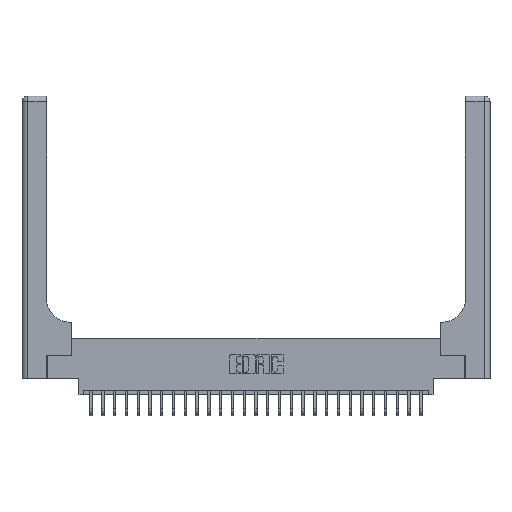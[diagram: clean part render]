
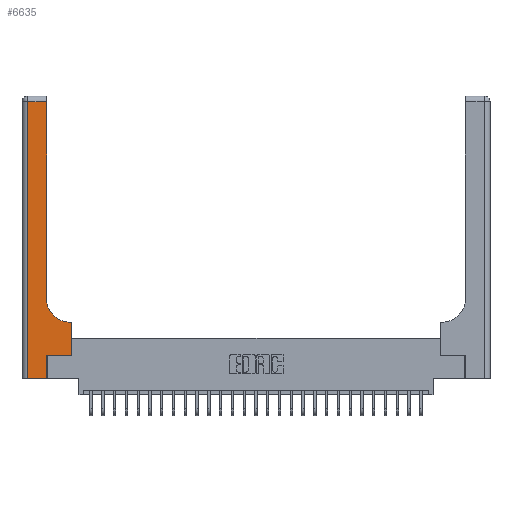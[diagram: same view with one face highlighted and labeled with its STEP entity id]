
A CAD part, top view. The second image highlights one B-rep face of the part: STEP entity #6635.
In plain terms, the highlighted planar face has unit normal (0, 0, 1).
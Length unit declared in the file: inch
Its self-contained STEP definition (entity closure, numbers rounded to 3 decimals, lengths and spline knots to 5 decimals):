
#686 = VECTOR ( 'NONE', #10712, 39.37008 ) ;
#997 = VERTEX_POINT ( 'NONE', #21001 ) ;
#1038 = EDGE_CURVE ( 'NONE', #25096, #25531, #8408, .T. ) ;
#1556 = LINE ( 'NONE', #10293, #5344 ) ;
#1730 = VERTEX_POINT ( 'NONE', #16154 ) ;
#1779 = CARTESIAN_POINT ( 'NONE',  ( 0., 2.94, 0.37 ) ) ;
#2214 = VERTEX_POINT ( 'NONE', #14119 ) ;
#2800 = ORIENTED_EDGE ( 'NONE', *, *, #14991, .T. ) ;
#3095 = VERTEX_POINT ( 'NONE', #4101 ) ;
#3140 = PLANE ( 'NONE',  #20049 ) ;
#3275 = FACE_OUTER_BOUND ( 'NONE', #4029, .T. ) ;
#4029 = EDGE_LOOP ( 'NONE', ( #19312, #25460, #20904, #24390, #14904, #2800, #17983, #15083, #19964 ) ) ;
#4101 = CARTESIAN_POINT ( 'NONE',  ( 0.06, 0., 0.37 ) ) ;
#4156 = DIRECTION ( 'NONE',  ( 0., 1., 0. ) ) ;
#4388 = VECTOR ( 'NONE', #26539, 39.37008 ) ;
#4410 = CARTESIAN_POINT ( 'NONE',  ( 0.06, 3., 0.37 ) ) ;
#4793 = CARTESIAN_POINT ( 'NONE',  ( 0.26, 0.85, 0.37 ) ) ;
#5344 = VECTOR ( 'NONE', #25563, 39.37008 ) ;
#5503 = VECTOR ( 'NONE', #4156, 39.37008 ) ;
#6266 = DIRECTION ( 'NONE',  ( 0., -1., 0. ) ) ;
#6635 = ADVANCED_FACE ( 'NONE', ( #3275 ), #3140, .F. ) ;
#8408 = LINE ( 'NONE', #23698, #686 ) ;
#8891 = LINE ( 'NONE', #23746, #5503 ) ;
#9444 = DIRECTION ( 'NONE',  ( 0., 0., -1. ) ) ;
#9636 = CARTESIAN_POINT ( 'NONE',  ( 0.51, 0.6, 0.37 ) ) ;
#10293 = CARTESIAN_POINT ( 'NONE',  ( 0.26, 0.6, 0.37 ) ) ;
#10712 = DIRECTION ( 'NONE',  ( 0., 1., 0. ) ) ;
#10732 = LINE ( 'NONE', #4410, #17349 ) ;
#10798 = EDGE_CURVE ( 'NONE', #13868, #2214, #25357, .T. ) ;
#11326 = DIRECTION ( 'NONE',  ( 1., 0., 0. ) ) ;
#11438 = EDGE_CURVE ( 'NONE', #997, #3095, #10732, .T. ) ;
#11492 = VECTOR ( 'NONE', #11326, 39.37008 ) ;
#12729 = LINE ( 'NONE', #21427, #4388 ) ;
#13023 = VECTOR ( 'NONE', #18801, 39.37008 ) ;
#13868 = VERTEX_POINT ( 'NONE', #14783 ) ;
#13890 = LINE ( 'NONE', #17619, #11492 ) ;
#14119 = CARTESIAN_POINT ( 'NONE',  ( 0.528, 0.6, 0.37 ) ) ;
#14783 = CARTESIAN_POINT ( 'NONE',  ( 0.528, 0.25, 0.37 ) ) ;
#14904 = ORIENTED_EDGE ( 'NONE', *, *, #24160, .T. ) ;
#14991 = EDGE_CURVE ( 'NONE', #17578, #13868, #12729, .T. ) ;
#15025 = DIRECTION ( 'NONE',  ( 0., 0., -1. ) ) ;
#15083 = ORIENTED_EDGE ( 'NONE', *, *, #16241, .T. ) ;
#15337 = DIRECTION ( 'NONE',  ( -1., 0., 0. ) ) ;
#15440 = AXIS2_PLACEMENT_3D ( 'NONE', #21445, #15025, #25856 ) ;
#16154 = CARTESIAN_POINT ( 'NONE',  ( 0.265, 0., 0.37 ) ) ;
#16241 = EDGE_CURVE ( 'NONE', #2214, #19268, #1556, .T. ) ;
#16524 = CARTESIAN_POINT ( 'NONE',  ( 0.528, 0.25, 0.37 ) ) ;
#17349 = VECTOR ( 'NONE', #6266, 39.37008 ) ;
#17578 = VERTEX_POINT ( 'NONE', #25722 ) ;
#17619 = CARTESIAN_POINT ( 'NONE',  ( 0., 0., 0.37 ) ) ;
#17983 = ORIENTED_EDGE ( 'NONE', *, *, #10798, .T. ) ;
#18039 = CARTESIAN_POINT ( 'NONE',  ( 0.26, 2.94, 0.37 ) ) ;
#18579 = EDGE_CURVE ( 'NONE', #19268, #25096, #19078, .T. ) ;
#18801 = DIRECTION ( 'NONE',  ( 0., 1., 0. ) ) ;
#19078 = CIRCLE ( 'NONE', #15440, 0.25 ) ;
#19255 = VECTOR ( 'NONE', #15337, 39.37008 ) ;
#19268 = VERTEX_POINT ( 'NONE', #9636 ) ;
#19312 = ORIENTED_EDGE ( 'NONE', *, *, #1038, .T. ) ;
#19964 = ORIENTED_EDGE ( 'NONE', *, *, #18579, .T. ) ;
#20049 = AXIS2_PLACEMENT_3D ( 'NONE', #25000, #9444, #22578 ) ;
#20904 = ORIENTED_EDGE ( 'NONE', *, *, #11438, .T. ) ;
#21001 = CARTESIAN_POINT ( 'NONE',  ( 0.06, 2.94, 0.37 ) ) ;
#21427 = CARTESIAN_POINT ( 'NONE',  ( 0.265, 0.25, 0.37 ) ) ;
#21445 = CARTESIAN_POINT ( 'NONE',  ( 0.51, 0.85, 0.37 ) ) ;
#22042 = LINE ( 'NONE', #1779, #19255 ) ;
#22578 = DIRECTION ( 'NONE',  ( -1., 0., 0. ) ) ;
#22997 = EDGE_CURVE ( 'NONE', #3095, #1730, #13890, .T. ) ;
#23698 = CARTESIAN_POINT ( 'NONE',  ( 0.26, 3., 0.37 ) ) ;
#23746 = CARTESIAN_POINT ( 'NONE',  ( 0.265, 0., 0.37 ) ) ;
#24160 = EDGE_CURVE ( 'NONE', #1730, #17578, #8891, .T. ) ;
#24390 = ORIENTED_EDGE ( 'NONE', *, *, #22997, .T. ) ;
#25000 = CARTESIAN_POINT ( 'NONE',  ( 0., 3., 0.37 ) ) ;
#25096 = VERTEX_POINT ( 'NONE', #4793 ) ;
#25313 = EDGE_CURVE ( 'NONE', #25531, #997, #22042, .T. ) ;
#25357 = LINE ( 'NONE', #16524, #13023 ) ;
#25460 = ORIENTED_EDGE ( 'NONE', *, *, #25313, .T. ) ;
#25531 = VERTEX_POINT ( 'NONE', #18039 ) ;
#25563 = DIRECTION ( 'NONE',  ( -1., 0., 0. ) ) ;
#25722 = CARTESIAN_POINT ( 'NONE',  ( 0.265, 0.25, 0.37 ) ) ;
#25856 = DIRECTION ( 'NONE',  ( 1., 0., 0. ) ) ;
#26539 = DIRECTION ( 'NONE',  ( 1., 0., 0. ) ) ;
